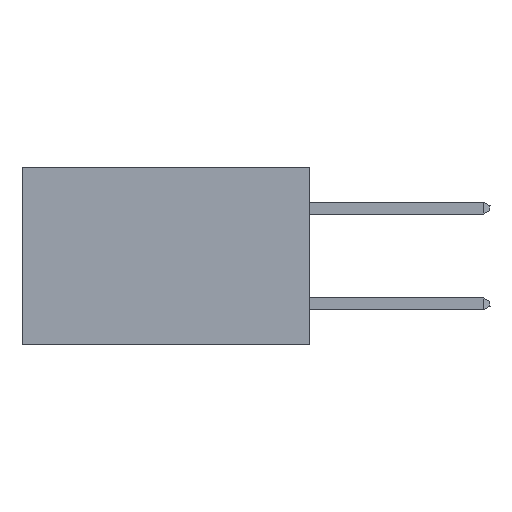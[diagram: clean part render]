
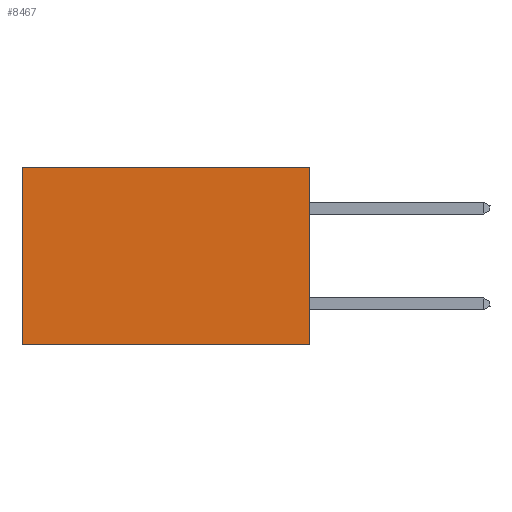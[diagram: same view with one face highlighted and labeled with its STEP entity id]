
A CAD part, left-side view. The second image highlights one B-rep face of the part: STEP entity #8467.
In plain terms, the highlighted planar face has unit normal (-1, 0, 0).
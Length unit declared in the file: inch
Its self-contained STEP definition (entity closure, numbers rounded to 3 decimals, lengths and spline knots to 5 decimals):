
#678 = CARTESIAN_POINT ( 'NONE',  ( 0.2875, 0., -0.37 ) ) ;
#1394 = DIRECTION ( 'NONE',  ( 1., 0., 0. ) ) ;
#2239 = LINE ( 'NONE', #28703, #22489 ) ;
#2391 = VERTEX_POINT ( 'NONE', #18594 ) ;
#3002 = DIRECTION ( 'NONE',  ( 0., 1., 0. ) ) ;
#3610 = DIRECTION ( 'NONE',  ( 0., 0., -1. ) ) ;
#4031 = EDGE_CURVE ( 'NONE', #2391, #14055, #4395, .T. ) ;
#4395 = LINE ( 'NONE', #31288, #22626 ) ;
#5269 = CARTESIAN_POINT ( 'NONE',  ( 0.2875, 0.6, -0.37 ) ) ;
#5896 = ORIENTED_EDGE ( 'NONE', *, *, #8096, .T. ) ;
#7485 = ORIENTED_EDGE ( 'NONE', *, *, #13983, .F. ) ;
#8096 = EDGE_CURVE ( 'NONE', #31098, #2391, #13254, .T. ) ;
#8467 = ADVANCED_FACE ( 'NONE', ( #30563 ), #31905, .F. ) ;
#8604 = ORIENTED_EDGE ( 'NONE', *, *, #4031, .T. ) ;
#8626 = ORIENTED_EDGE ( 'NONE', *, *, #23518, .F. ) ;
#10491 = DIRECTION ( 'NONE',  ( 0., 0., -1. ) ) ;
#10518 = CARTESIAN_POINT ( 'NONE',  ( 0.2875, 0., 0. ) ) ;
#11537 = CARTESIAN_POINT ( 'NONE',  ( 0.2875, 0., 0. ) ) ;
#13109 = DIRECTION ( 'NONE',  ( 0., 1., 0. ) ) ;
#13254 = LINE ( 'NONE', #10518, #21376 ) ;
#13983 = EDGE_CURVE ( 'NONE', #26742, #14055, #2239, .T. ) ;
#14055 = VERTEX_POINT ( 'NONE', #5269 ) ;
#15569 = DIRECTION ( 'NONE',  ( 0., 0., -1. ) ) ;
#16565 = EDGE_LOOP ( 'NONE', ( #8604, #7485, #8626, #5896 ) ) ;
#18594 = CARTESIAN_POINT ( 'NONE',  ( 0.2875, 0.6, 0. ) ) ;
#19608 = LINE ( 'NONE', #23646, #29188 ) ;
#21376 = VECTOR ( 'NONE', #13109, 39.37008 ) ;
#22489 = VECTOR ( 'NONE', #3002, 39.37008 ) ;
#22626 = VECTOR ( 'NONE', #10491, 39.37008 ) ;
#23518 = EDGE_CURVE ( 'NONE', #31098, #26742, #19608, .T. ) ;
#23646 = CARTESIAN_POINT ( 'NONE',  ( 0.2875, 0., 0. ) ) ;
#26594 = CARTESIAN_POINT ( 'NONE',  ( 0.2875, 0., 0. ) ) ;
#26742 = VERTEX_POINT ( 'NONE', #678 ) ;
#28031 = AXIS2_PLACEMENT_3D ( 'NONE', #11537, #1394, #3610 ) ;
#28703 = CARTESIAN_POINT ( 'NONE',  ( 0.2875, 0., -0.37 ) ) ;
#29188 = VECTOR ( 'NONE', #15569, 39.37008 ) ;
#30563 = FACE_OUTER_BOUND ( 'NONE', #16565, .T. ) ;
#31098 = VERTEX_POINT ( 'NONE', #26594 ) ;
#31288 = CARTESIAN_POINT ( 'NONE',  ( 0.2875, 0.6, 0. ) ) ;
#31905 = PLANE ( 'NONE',  #28031 ) ;
